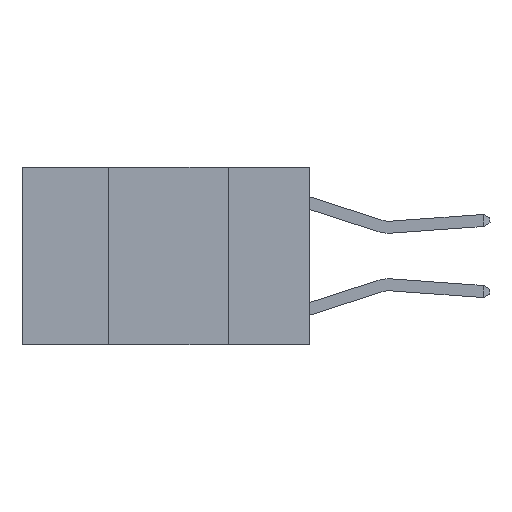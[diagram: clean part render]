
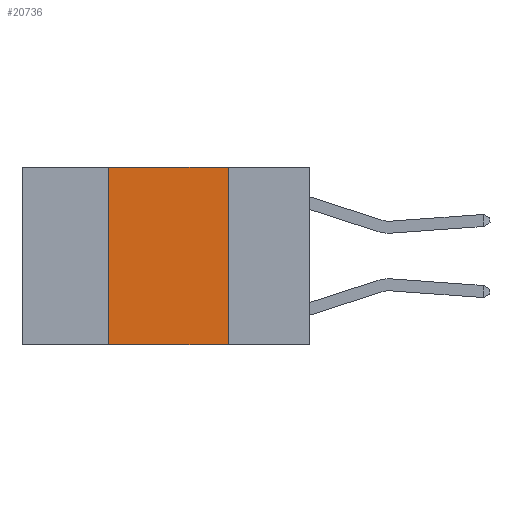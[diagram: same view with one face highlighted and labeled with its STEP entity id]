
A CAD part, left-side view. The second image highlights one B-rep face of the part: STEP entity #20736.
In plain terms, the highlighted planar face has unit normal (-1, 0, 0).
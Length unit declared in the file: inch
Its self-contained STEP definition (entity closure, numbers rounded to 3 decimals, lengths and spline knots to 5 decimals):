
#377 = EDGE_CURVE ( 'NONE', #1474, #19686, #8963, .T. ) ;
#1037 = FACE_OUTER_BOUND ( 'NONE', #11459, .T. ) ;
#1426 = AXIS2_PLACEMENT_3D ( 'NONE', #17130, #22819, #11476 ) ;
#1474 = VERTEX_POINT ( 'NONE', #6962 ) ;
#3336 = ORIENTED_EDGE ( 'NONE', *, *, #18090, .F. ) ;
#4780 = CARTESIAN_POINT ( 'NONE',  ( 0., 0.17, 0. ) ) ;
#4919 = LINE ( 'NONE', #7001, #23827 ) ;
#6388 = DIRECTION ( 'NONE',  ( 0., -1., 0. ) ) ;
#6717 = CARTESIAN_POINT ( 'NONE',  ( 0., 0.6, -0.37 ) ) ;
#6962 = CARTESIAN_POINT ( 'NONE',  ( 0., 0.42, -0.37 ) ) ;
#7001 = CARTESIAN_POINT ( 'NONE',  ( 0., 0.17, 0. ) ) ;
#8337 = LINE ( 'NONE', #21042, #17819 ) ;
#8903 = DIRECTION ( 'NONE',  ( 0., 0., -1. ) ) ;
#8963 = LINE ( 'NONE', #6717, #23461 ) ;
#9591 = PLANE ( 'NONE',  #1426 ) ;
#11459 = EDGE_LOOP ( 'NONE', ( #12226, #3336, #18013, #13163 ) ) ;
#11476 = DIRECTION ( 'NONE',  ( 0., 0., -1. ) ) ;
#11532 = VERTEX_POINT ( 'NONE', #4780 ) ;
#12226 = ORIENTED_EDGE ( 'NONE', *, *, #21231, .F. ) ;
#12641 = CARTESIAN_POINT ( 'NONE',  ( 0., 0.42, 0. ) ) ;
#13163 = ORIENTED_EDGE ( 'NONE', *, *, #377, .T. ) ;
#13733 = VECTOR ( 'NONE', #15946, 39.37008 ) ;
#14960 = VERTEX_POINT ( 'NONE', #12641 ) ;
#15946 = DIRECTION ( 'NONE',  ( 0., -1., 0. ) ) ;
#17130 = CARTESIAN_POINT ( 'NONE',  ( 0., 0.6, 0. ) ) ;
#17330 = DIRECTION ( 'NONE',  ( 0., 0., 1. ) ) ;
#17819 = VECTOR ( 'NONE', #17330, 39.37008 ) ;
#18013 = ORIENTED_EDGE ( 'NONE', *, *, #23731, .F. ) ;
#18090 = EDGE_CURVE ( 'NONE', #14960, #11532, #18176, .T. ) ;
#18176 = LINE ( 'NONE', #19727, #13733 ) ;
#18607 = CARTESIAN_POINT ( 'NONE',  ( 0., 0.17, -0.37 ) ) ;
#19686 = VERTEX_POINT ( 'NONE', #18607 ) ;
#19727 = CARTESIAN_POINT ( 'NONE',  ( 0., 0.6, 0. ) ) ;
#20736 = ADVANCED_FACE ( 'NONE', ( #1037 ), #9591, .F. ) ;
#21042 = CARTESIAN_POINT ( 'NONE',  ( 0., 0.42, 0. ) ) ;
#21231 = EDGE_CURVE ( 'NONE', #11532, #19686, #4919, .T. ) ;
#22819 = DIRECTION ( 'NONE',  ( 1., 0., 0. ) ) ;
#23461 = VECTOR ( 'NONE', #6388, 39.37008 ) ;
#23731 = EDGE_CURVE ( 'NONE', #1474, #14960, #8337, .T. ) ;
#23827 = VECTOR ( 'NONE', #8903, 39.37008 ) ;
